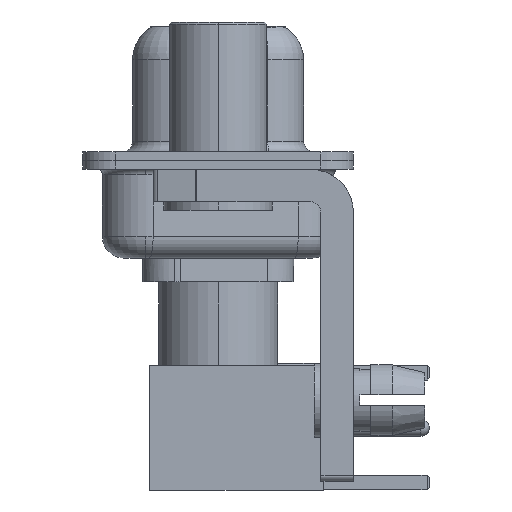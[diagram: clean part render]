
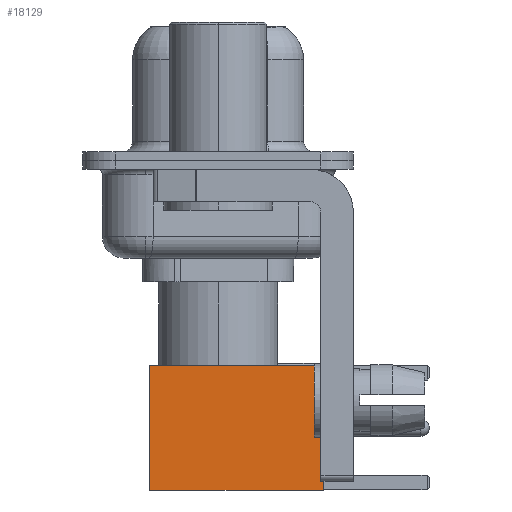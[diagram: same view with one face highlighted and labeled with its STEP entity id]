
A CAD part, left-side view. The second image highlights one B-rep face of the part: STEP entity #18129.
In plain terms, the highlighted face is planar.
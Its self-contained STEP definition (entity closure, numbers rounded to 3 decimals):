
#828 = EDGE_CURVE ( 'NONE', #4177, #3949, #6527, .T. ) ;
#998 = ORIENTED_EDGE ( 'NONE', *, *, #11960, .T. ) ;
#1161 = ORIENTED_EDGE ( 'NONE', *, *, #828, .F. ) ;
#2201 = VERTEX_POINT ( 'NONE', #15934 ) ;
#3519 = DIRECTION ( 'NONE',  ( -1., 0., 0. ) ) ;
#3706 = CARTESIAN_POINT ( 'NONE',  ( -2.875, 2.875, 8. ) ) ;
#3949 = VERTEX_POINT ( 'NONE', #13595 ) ;
#4177 = VERTEX_POINT ( 'NONE', #3706 ) ;
#5341 = VECTOR ( 'NONE', #17149, 1000. ) ;
#5732 = VECTOR ( 'NONE', #6293, 1000. ) ;
#5883 = VECTOR ( 'NONE', #3519, 1000. ) ;
#6293 = DIRECTION ( 'NONE',  ( 0., 0., -1. ) ) ;
#6497 = EDGE_CURVE ( 'NONE', #12796, #4177, #20429, .T. ) ;
#6527 = LINE ( 'NONE', #10033, #14369 ) ;
#8057 = CARTESIAN_POINT ( 'NONE',  ( 2.875, 2.875, 0. ) ) ;
#9120 = CARTESIAN_POINT ( 'NONE',  ( 0., 2.875, 0. ) ) ;
#9159 = FACE_OUTER_BOUND ( 'NONE', #10413, .T. ) ;
#9451 = AXIS2_PLACEMENT_3D ( 'NONE', #13409, #22838, #13283 ) ;
#10033 = CARTESIAN_POINT ( 'NONE',  ( -2.875, 2.875, 0. ) ) ;
#10413 = EDGE_LOOP ( 'NONE', ( #998, #21348, #1161, #17273 ) ) ;
#11794 = LINE ( 'NONE', #8057, #5732 ) ;
#11960 = EDGE_CURVE ( 'NONE', #12796, #2201, #11794, .T. ) ;
#12131 = EDGE_CURVE ( 'NONE', #2201, #3949, #22679, .T. ) ;
#12796 = VERTEX_POINT ( 'NONE', #17429 ) ;
#13283 = DIRECTION ( 'NONE',  ( 0., 0., 1. ) ) ;
#13409 = CARTESIAN_POINT ( 'NONE',  ( 2.875, 2.875, 0. ) ) ;
#13595 = CARTESIAN_POINT ( 'NONE',  ( -2.875, 2.875, 0. ) ) ;
#13788 = DIRECTION ( 'NONE',  ( 0., 0., -1. ) ) ;
#14369 = VECTOR ( 'NONE', #13788, 1000. ) ;
#15934 = CARTESIAN_POINT ( 'NONE',  ( 2.875, 2.875, 0. ) ) ;
#17149 = DIRECTION ( 'NONE',  ( -1., 0., 0. ) ) ;
#17273 = ORIENTED_EDGE ( 'NONE', *, *, #6497, .F. ) ;
#17429 = CARTESIAN_POINT ( 'NONE',  ( 2.875, 2.875, 8. ) ) ;
#18129 = ADVANCED_FACE ( 'NONE', ( #9159 ), #18818, .T. ) ;
#18818 = PLANE ( 'NONE',  #9451 ) ;
#20429 = LINE ( 'NONE', #20554, #5883 ) ;
#20554 = CARTESIAN_POINT ( 'NONE',  ( 0., 2.875, 8. ) ) ;
#21348 = ORIENTED_EDGE ( 'NONE', *, *, #12131, .T. ) ;
#22679 = LINE ( 'NONE', #9120, #5341 ) ;
#22838 = DIRECTION ( 'NONE',  ( 0., 1., 0. ) ) ;
